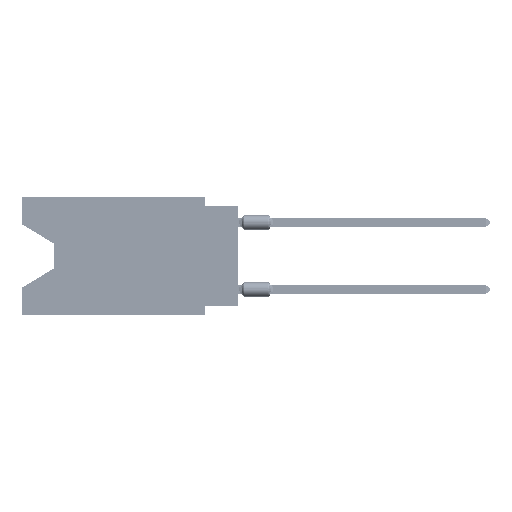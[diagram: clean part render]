
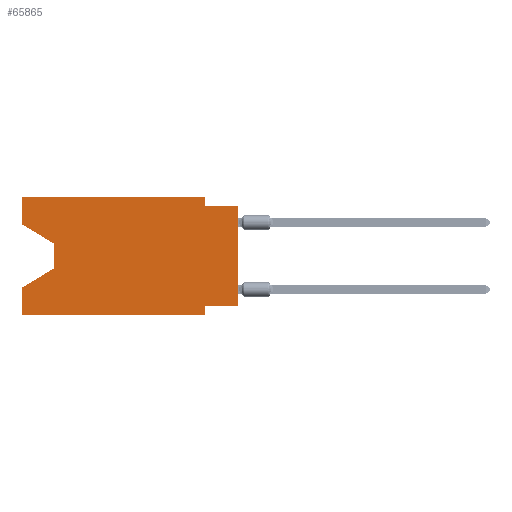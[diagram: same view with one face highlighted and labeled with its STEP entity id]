
A CAD part, left-side view. The second image highlights one B-rep face of the part: STEP entity #65865.
In plain terms, the highlighted planar face has unit normal (-1, 0, 0).
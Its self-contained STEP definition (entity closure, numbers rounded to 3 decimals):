
#1654 = ORIENTED_EDGE ( 'NONE', *, *, #10251, .F. ) ;
#1942 = CARTESIAN_POINT ( 'NONE',  ( 0., 16.383, -2.038 ) ) ;
#2127 = CARTESIAN_POINT ( 'NONE',  ( 0., 2.54, -8.89 ) ) ;
#2359 = CARTESIAN_POINT ( 'NONE',  ( 0., 16.383, -8.89 ) ) ;
#3789 = LINE ( 'NONE', #29442, #9258 ) ;
#4164 = VECTOR ( 'NONE', #62847, 1000. ) ;
#4807 = EDGE_CURVE ( 'NONE', #47854, #5455, #27476, .T. ) ;
#5455 = VERTEX_POINT ( 'NONE', #23540 ) ;
#5833 = CARTESIAN_POINT ( 'NONE',  ( 0., 13.97, -5.385 ) ) ;
#7596 = DIRECTION ( 'NONE',  ( 0., 1., 0. ) ) ;
#9063 = VECTOR ( 'NONE', #52911, 1000. ) ;
#9258 = VECTOR ( 'NONE', #60972, 1000. ) ;
#9262 = CARTESIAN_POINT ( 'NONE',  ( 0., 16.383, 0. ) ) ;
#9793 = VERTEX_POINT ( 'NONE', #2359 ) ;
#10251 = EDGE_CURVE ( 'NONE', #13003, #12386, #3789, .T. ) ;
#10807 = AXIS2_PLACEMENT_3D ( 'NONE', #9262, #66025, #21878 ) ;
#10977 = LINE ( 'NONE', #29485, #27054 ) ;
#11266 = CARTESIAN_POINT ( 'NONE',  ( 0., 2.54, -8.255 ) ) ;
#11468 = DIRECTION ( 'NONE',  ( 0., 0., -1. ) ) ;
#12386 = VERTEX_POINT ( 'NONE', #52493 ) ;
#13003 = VERTEX_POINT ( 'NONE', #1942 ) ;
#13902 = CARTESIAN_POINT ( 'NONE',  ( 0., 0., -8.255 ) ) ;
#14539 = DIRECTION ( 'NONE',  ( 0., 0., 1. ) ) ;
#16530 = LINE ( 'NONE', #69044, #41926 ) ;
#17208 = EDGE_CURVE ( 'NONE', #33081, #5455, #47315, .T. ) ;
#17390 = CARTESIAN_POINT ( 'NONE',  ( 0., 16.383, -6.852 ) ) ;
#18451 = DIRECTION ( 'NONE',  ( 0., 0.855, -0.519 ) ) ;
#18871 = LINE ( 'NONE', #5833, #75903 ) ;
#19718 = CARTESIAN_POINT ( 'NONE',  ( 0., 2.54, 0. ) ) ;
#19922 = VERTEX_POINT ( 'NONE', #2127 ) ;
#20269 = ORIENTED_EDGE ( 'NONE', *, *, #59855, .T. ) ;
#20966 = LINE ( 'NONE', #26019, #9063 ) ;
#21036 = LINE ( 'NONE', #13902, #49802 ) ;
#21878 = DIRECTION ( 'NONE',  ( 0., 0., -1. ) ) ;
#23123 = EDGE_CURVE ( 'NONE', #80649, #19922, #24520, .T. ) ;
#23147 = EDGE_CURVE ( 'NONE', #33081, #80649, #21036, .T. ) ;
#23540 = CARTESIAN_POINT ( 'NONE',  ( 0., 0., -0.635 ) ) ;
#24157 = ORIENTED_EDGE ( 'NONE', *, *, #4807, .F. ) ;
#24520 = LINE ( 'NONE', #50179, #59375 ) ;
#26019 = CARTESIAN_POINT ( 'NONE',  ( 0., 16.383, 0. ) ) ;
#27054 = VECTOR ( 'NONE', #36204, 1000. ) ;
#27476 = LINE ( 'NONE', #27887, #28870 ) ;
#27887 = CARTESIAN_POINT ( 'NONE',  ( 0., 0., -0.635 ) ) ;
#28537 = EDGE_CURVE ( 'NONE', #9793, #19922, #36403, .T. ) ;
#28870 = VECTOR ( 'NONE', #53524, 1000. ) ;
#29377 = EDGE_CURVE ( 'NONE', #12386, #66174, #10977, .T. ) ;
#29442 = CARTESIAN_POINT ( 'NONE',  ( 0., 16.383, 0. ) ) ;
#29485 = CARTESIAN_POINT ( 'NONE',  ( 0., 16.383, 0. ) ) ;
#30387 = ORIENTED_EDGE ( 'NONE', *, *, #29377, .F. ) ;
#32214 = LINE ( 'NONE', #57855, #63683 ) ;
#32359 = ORIENTED_EDGE ( 'NONE', *, *, #23147, .F. ) ;
#33081 = VERTEX_POINT ( 'NONE', #33858 ) ;
#33858 = CARTESIAN_POINT ( 'NONE',  ( 0., 0., -8.255 ) ) ;
#34739 = ORIENTED_EDGE ( 'NONE', *, *, #17208, .T. ) ;
#34907 = FACE_OUTER_BOUND ( 'NONE', #65642, .T. ) ;
#35250 = VERTEX_POINT ( 'NONE', #62819 ) ;
#36204 = DIRECTION ( 'NONE',  ( 0., -1., 0. ) ) ;
#36403 = LINE ( 'NONE', #82618, #4164 ) ;
#38136 = CARTESIAN_POINT ( 'NONE',  ( 0., 2.54, -0.635 ) ) ;
#39089 = ORIENTED_EDGE ( 'NONE', *, *, #42054, .F. ) ;
#39098 = EDGE_CURVE ( 'NONE', #35250, #82161, #69677, .T. ) ;
#39668 = ORIENTED_EDGE ( 'NONE', *, *, #48447, .F. ) ;
#41090 = VECTOR ( 'NONE', #14539, 1000. ) ;
#41926 = VECTOR ( 'NONE', #11468, 1000. ) ;
#42054 = EDGE_CURVE ( 'NONE', #66174, #47854, #16530, .T. ) ;
#44337 = EDGE_CURVE ( 'NONE', #13003, #35250, #32214, .T. ) ;
#46754 = ORIENTED_EDGE ( 'NONE', *, *, #44337, .T. ) ;
#47315 = LINE ( 'NONE', #67028, #41090 ) ;
#47854 = VERTEX_POINT ( 'NONE', #38136 ) ;
#48447 = EDGE_CURVE ( 'NONE', #9793, #62630, #20966, .T. ) ;
#49802 = VECTOR ( 'NONE', #7596, 1000. ) ;
#50179 = CARTESIAN_POINT ( 'NONE',  ( 0., 2.54, -8.89 ) ) ;
#51616 = DIRECTION ( 'NONE',  ( 0., 0., -1. ) ) ;
#52493 = CARTESIAN_POINT ( 'NONE',  ( 0., 16.383, 0. ) ) ;
#52911 = DIRECTION ( 'NONE',  ( 0., 0., 1. ) ) ;
#53524 = DIRECTION ( 'NONE',  ( 0., -1., 0. ) ) ;
#54051 = ORIENTED_EDGE ( 'NONE', *, *, #23123, .F. ) ;
#57406 = VECTOR ( 'NONE', #51616, 1000. ) ;
#57855 = CARTESIAN_POINT ( 'NONE',  ( 0., 16.383, -2.038 ) ) ;
#58184 = ORIENTED_EDGE ( 'NONE', *, *, #39098, .T. ) ;
#59375 = VECTOR ( 'NONE', #75810, 1000. ) ;
#59855 = EDGE_CURVE ( 'NONE', #82161, #62630, #18871, .T. ) ;
#60972 = DIRECTION ( 'NONE',  ( 0., 0., 1. ) ) ;
#62630 = VERTEX_POINT ( 'NONE', #17390 ) ;
#62819 = CARTESIAN_POINT ( 'NONE',  ( 0., 13.97, -3.505 ) ) ;
#62847 = DIRECTION ( 'NONE',  ( 0., -1., 0. ) ) ;
#63683 = VECTOR ( 'NONE', #64563, 1000. ) ;
#64563 = DIRECTION ( 'NONE',  ( 0., -0.855, -0.519 ) ) ;
#65642 = EDGE_LOOP ( 'NONE', ( #46754, #58184, #20269, #39668, #75019, #54051, #32359, #34739, #24157, #39089, #30387, #1654 ) ) ;
#65865 = ADVANCED_FACE ( 'NONE', ( #34907 ), #71511, .F. ) ;
#66025 = DIRECTION ( 'NONE',  ( 1., 0., 0. ) ) ;
#66174 = VERTEX_POINT ( 'NONE', #19718 ) ;
#67028 = CARTESIAN_POINT ( 'NONE',  ( 0., 0., 0. ) ) ;
#69044 = CARTESIAN_POINT ( 'NONE',  ( 0., 2.54, 0. ) ) ;
#69677 = LINE ( 'NONE', #82298, #57406 ) ;
#71511 = PLANE ( 'NONE',  #10807 ) ;
#75019 = ORIENTED_EDGE ( 'NONE', *, *, #28537, .T. ) ;
#75810 = DIRECTION ( 'NONE',  ( 0., 0., -1. ) ) ;
#75903 = VECTOR ( 'NONE', #18451, 1000. ) ;
#76525 = CARTESIAN_POINT ( 'NONE',  ( 0., 13.97, -5.385 ) ) ;
#80649 = VERTEX_POINT ( 'NONE', #11266 ) ;
#82161 = VERTEX_POINT ( 'NONE', #76525 ) ;
#82298 = CARTESIAN_POINT ( 'NONE',  ( 0., 13.97, -3.505 ) ) ;
#82618 = CARTESIAN_POINT ( 'NONE',  ( 0., 16.383, -8.89 ) ) ;
